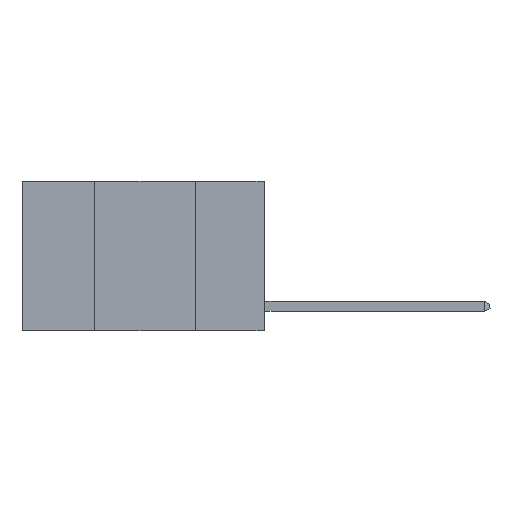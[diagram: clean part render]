
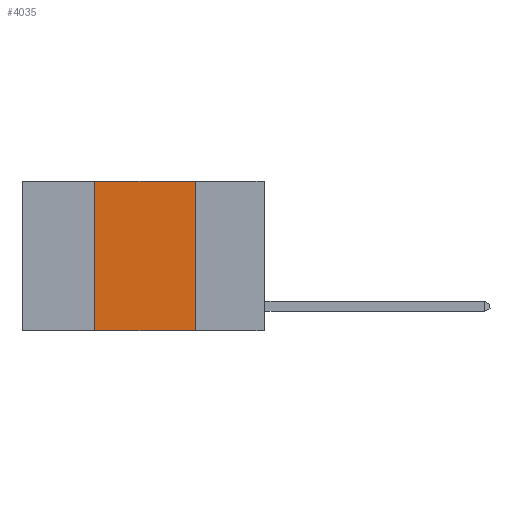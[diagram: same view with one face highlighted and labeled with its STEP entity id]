
A CAD part, left-side view. The second image highlights one B-rep face of the part: STEP entity #4035.
In plain terms, the highlighted planar face has unit normal (-1, 0, 0).
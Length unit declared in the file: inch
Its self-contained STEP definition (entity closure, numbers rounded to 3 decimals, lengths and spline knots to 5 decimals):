
#712 = CARTESIAN_POINT ( 'NONE',  ( 0., 0.6, 0. ) ) ;
#713 = EDGE_CURVE ( 'NONE', #1733, #5507, #2521, .T. ) ;
#855 = EDGE_CURVE ( 'NONE', #5507, #5926, #1579, .T. ) ;
#1046 = VECTOR ( 'NONE', #7834, 39.37008 ) ;
#1109 = CARTESIAN_POINT ( 'NONE',  ( 0., 0.17, -0.37 ) ) ;
#1271 = VECTOR ( 'NONE', #1960, 39.37008 ) ;
#1341 = LINE ( 'NONE', #7770, #1271 ) ;
#1553 = CARTESIAN_POINT ( 'NONE',  ( 0., 0.42, 0. ) ) ;
#1579 = LINE ( 'NONE', #4126, #5679 ) ;
#1733 = VERTEX_POINT ( 'NONE', #1553 ) ;
#1960 = DIRECTION ( 'NONE',  ( 0., -1., 0. ) ) ;
#2521 = LINE ( 'NONE', #712, #7639 ) ;
#2775 = CARTESIAN_POINT ( 'NONE',  ( 0., 0.42, 0. ) ) ;
#3076 = EDGE_CURVE ( 'NONE', #3786, #1733, #6043, .T. ) ;
#3786 = VERTEX_POINT ( 'NONE', #7606 ) ;
#4029 = ORIENTED_EDGE ( 'NONE', *, *, #855, .F. ) ;
#4035 = ADVANCED_FACE ( 'NONE', ( #6027 ), #5356, .F. ) ;
#4126 = CARTESIAN_POINT ( 'NONE',  ( 0., 0.17, 0. ) ) ;
#4683 = CARTESIAN_POINT ( 'NONE',  ( 0., 0.6, 0. ) ) ;
#4719 = AXIS2_PLACEMENT_3D ( 'NONE', #4683, #7238, #7322 ) ;
#5356 = PLANE ( 'NONE',  #4719 ) ;
#5507 = VERTEX_POINT ( 'NONE', #5618 ) ;
#5618 = CARTESIAN_POINT ( 'NONE',  ( 0., 0.17, 0. ) ) ;
#5679 = VECTOR ( 'NONE', #6645, 39.37008 ) ;
#5755 = DIRECTION ( 'NONE',  ( 0., -1., 0. ) ) ;
#5926 = VERTEX_POINT ( 'NONE', #1109 ) ;
#5966 = ORIENTED_EDGE ( 'NONE', *, *, #713, .F. ) ;
#6027 = FACE_OUTER_BOUND ( 'NONE', #6245, .T. ) ;
#6043 = LINE ( 'NONE', #2775, #1046 ) ;
#6067 = EDGE_CURVE ( 'NONE', #3786, #5926, #1341, .T. ) ;
#6206 = ORIENTED_EDGE ( 'NONE', *, *, #6067, .T. ) ;
#6245 = EDGE_LOOP ( 'NONE', ( #4029, #5966, #7175, #6206 ) ) ;
#6645 = DIRECTION ( 'NONE',  ( 0., 0., -1. ) ) ;
#7175 = ORIENTED_EDGE ( 'NONE', *, *, #3076, .F. ) ;
#7238 = DIRECTION ( 'NONE',  ( 1., 0., 0. ) ) ;
#7322 = DIRECTION ( 'NONE',  ( 0., 0., -1. ) ) ;
#7606 = CARTESIAN_POINT ( 'NONE',  ( 0., 0.42, -0.37 ) ) ;
#7639 = VECTOR ( 'NONE', #5755, 39.37008 ) ;
#7770 = CARTESIAN_POINT ( 'NONE',  ( 0., 0.6, -0.37 ) ) ;
#7834 = DIRECTION ( 'NONE',  ( 0., 0., 1. ) ) ;
